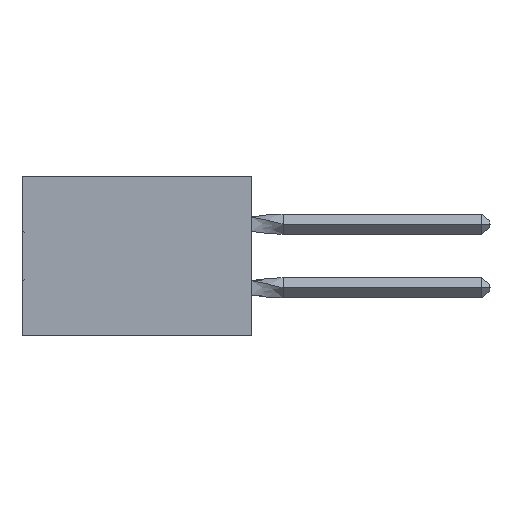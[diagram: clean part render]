
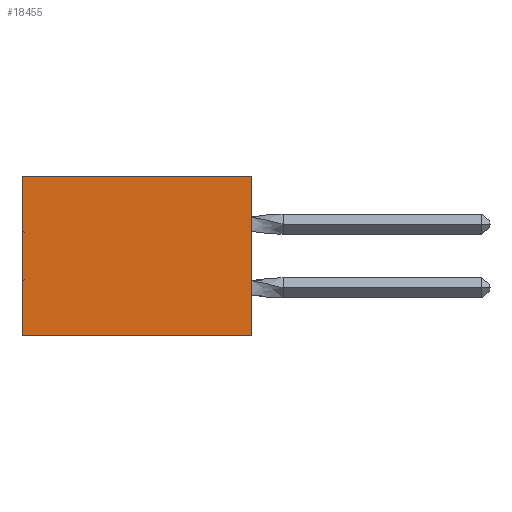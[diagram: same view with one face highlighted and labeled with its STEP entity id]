
A CAD part, left-side view. The second image highlights one B-rep face of the part: STEP entity #18455.
In plain terms, the highlighted planar face has unit normal (-1, 0, 0).
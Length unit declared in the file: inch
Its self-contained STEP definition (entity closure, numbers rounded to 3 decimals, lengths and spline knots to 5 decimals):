
#823 = ORIENTED_EDGE ( 'NONE', *, *, #13541, .F. ) ;
#1405 = VERTEX_POINT ( 'NONE', #22152 ) ;
#3145 = DIRECTION ( 'NONE',  ( 0., 1., 0. ) ) ;
#3218 = VECTOR ( 'NONE', #5245, 39.37008 ) ;
#3561 = AXIS2_PLACEMENT_3D ( 'NONE', #9114, #51338, #17286 ) ;
#3692 = CARTESIAN_POINT ( 'NONE',  ( 0.305, 0., -0.5 ) ) ;
#3749 = CARTESIAN_POINT ( 'NONE',  ( 0.305, 0., 0. ) ) ;
#5245 = DIRECTION ( 'NONE',  ( 0., 0., -1. ) ) ;
#7847 = LINE ( 'NONE', #13769, #3218 ) ;
#9114 = CARTESIAN_POINT ( 'NONE',  ( 0.305, 0., -0.5 ) ) ;
#9299 = PLANE ( 'NONE',  #3561 ) ;
#10618 = CARTESIAN_POINT ( 'NONE',  ( 0.305, 0., 0. ) ) ;
#10773 = VECTOR ( 'NONE', #22723, 39.37008 ) ;
#11168 = DIRECTION ( 'NONE',  ( 0., 1., 0. ) ) ;
#12106 = VECTOR ( 'NONE', #11168, 39.37008 ) ;
#13541 = EDGE_CURVE ( 'NONE', #33862, #24707, #41483, .T. ) ;
#13769 = CARTESIAN_POINT ( 'NONE',  ( 0.305, 0.72, -0.5 ) ) ;
#17286 = DIRECTION ( 'NONE',  ( 0., 0., -1. ) ) ;
#18125 = EDGE_CURVE ( 'NONE', #25562, #33862, #32693, .T. ) ;
#18455 = ADVANCED_FACE ( 'NONE', ( #36010 ), #9299, .F. ) ;
#20248 = EDGE_CURVE ( 'NONE', #1405, #24707, #7847, .T. ) ;
#22152 = CARTESIAN_POINT ( 'NONE',  ( 0.305, 0.72, 0. ) ) ;
#22723 = DIRECTION ( 'NONE',  ( 0., 0., -1. ) ) ;
#24707 = VERTEX_POINT ( 'NONE', #33821 ) ;
#25562 = VERTEX_POINT ( 'NONE', #3749 ) ;
#26793 = VECTOR ( 'NONE', #3145, 39.37008 ) ;
#30780 = CARTESIAN_POINT ( 'NONE',  ( 0.305, 0., -0.5 ) ) ;
#32660 = EDGE_LOOP ( 'NONE', ( #38794, #823, #46936, #34989 ) ) ;
#32693 = LINE ( 'NONE', #30780, #10773 ) ;
#33821 = CARTESIAN_POINT ( 'NONE',  ( 0.305, 0.72, -0.5 ) ) ;
#33862 = VERTEX_POINT ( 'NONE', #44631 ) ;
#34989 = ORIENTED_EDGE ( 'NONE', *, *, #49955, .T. ) ;
#36010 = FACE_OUTER_BOUND ( 'NONE', #32660, .T. ) ;
#38794 = ORIENTED_EDGE ( 'NONE', *, *, #20248, .T. ) ;
#41483 = LINE ( 'NONE', #3692, #26793 ) ;
#44631 = CARTESIAN_POINT ( 'NONE',  ( 0.305, 0., -0.5 ) ) ;
#45339 = LINE ( 'NONE', #10618, #12106 ) ;
#46936 = ORIENTED_EDGE ( 'NONE', *, *, #18125, .F. ) ;
#49955 = EDGE_CURVE ( 'NONE', #25562, #1405, #45339, .T. ) ;
#51338 = DIRECTION ( 'NONE',  ( 1., 0., 0. ) ) ;
